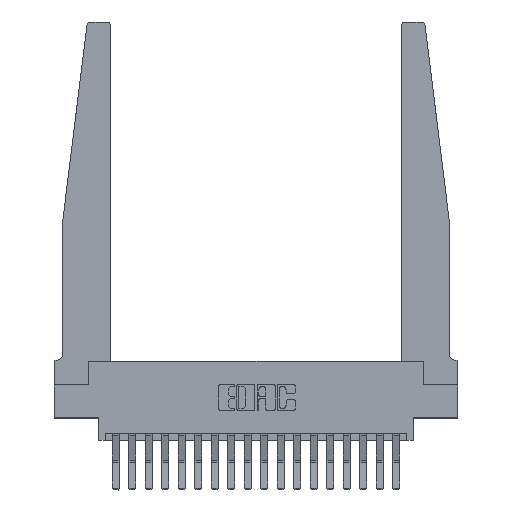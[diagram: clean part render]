
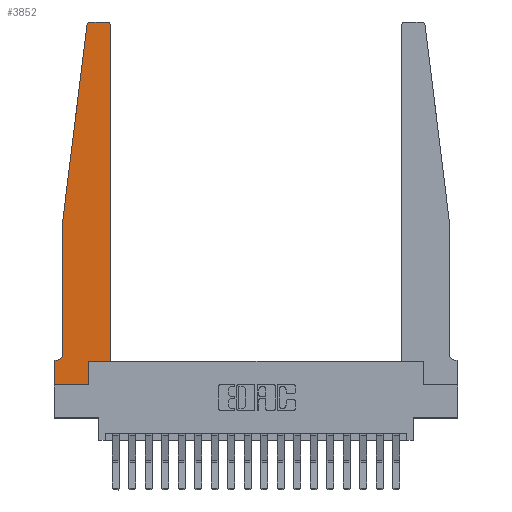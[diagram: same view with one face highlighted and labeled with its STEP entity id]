
A CAD part, top view. The second image highlights one B-rep face of the part: STEP entity #3852.
In plain terms, the highlighted planar face has unit normal (0, 0, 1).
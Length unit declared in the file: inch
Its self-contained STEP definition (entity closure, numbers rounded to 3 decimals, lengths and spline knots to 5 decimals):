
#74 = DIRECTION ( 'NONE',  ( 0., 1., 0. ) ) ;
#205 = DIRECTION ( 'NONE',  ( 0., 0., 1. ) ) ;
#353 = EDGE_LOOP ( 'NONE', ( #4655, #19632, #8052, #14852, #11743, #19731, #17841, #4805, #10594, #14451, #12872, #9959 ) ) ;
#477 = EDGE_CURVE ( 'NONE', #16946, #14493, #8638, .T. ) ;
#499 = CARTESIAN_POINT ( 'NONE',  ( 0.015, 0.2375, 0.37 ) ) ;
#650 = CIRCLE ( 'NONE', #15962, 0.03 ) ;
#971 = EDGE_CURVE ( 'NONE', #14493, #1321, #3538, .T. ) ;
#1109 = VECTOR ( 'NONE', #5097, 39.37008 ) ;
#1321 = VERTEX_POINT ( 'NONE', #9912 ) ;
#1363 = CARTESIAN_POINT ( 'NONE',  ( 0.065, 0.1875, 0.37 ) ) ;
#1855 = VECTOR ( 'NONE', #16621, 39.37008 ) ;
#2051 = DIRECTION ( 'NONE',  ( -1., 0., 0. ) ) ;
#2540 = CARTESIAN_POINT ( 'NONE',  ( 0., 0.1875, 0.37 ) ) ;
#3120 = CARTESIAN_POINT ( 'NONE',  ( 0.25, 2.75, 0.37 ) ) ;
#3167 = CARTESIAN_POINT ( 'NONE',  ( 0.425, 0.18, 0.37 ) ) ;
#3538 = CIRCLE ( 'NONE', #10757, 0.03 ) ;
#3852 = ADVANCED_FACE ( 'NONE', ( #19087 ), #6340, .T. ) ;
#3953 = CARTESIAN_POINT ( 'NONE',  ( 0., 0., 0.37 ) ) ;
#4562 = VERTEX_POINT ( 'NONE', #14441 ) ;
#4655 = ORIENTED_EDGE ( 'NONE', *, *, #477, .T. ) ;
#4674 = VECTOR ( 'NONE', #74, 39.37008 ) ;
#4805 = ORIENTED_EDGE ( 'NONE', *, *, #18043, .T. ) ;
#5097 = DIRECTION ( 'NONE',  ( 1., 0., 0. ) ) ;
#5315 = LINE ( 'NONE', #15316, #12548 ) ;
#5575 = DIRECTION ( 'NONE',  ( 0., 0., 1. ) ) ;
#5767 = DIRECTION ( 'NONE',  ( 0., -1., 0. ) ) ;
#5957 = LINE ( 'NONE', #7456, #1855 ) ;
#6118 = VECTOR ( 'NONE', #5767, 39.37008 ) ;
#6211 = VERTEX_POINT ( 'NONE', #19633 ) ;
#6285 = CARTESIAN_POINT ( 'NONE',  ( 0.2605, 0.18, 0.37 ) ) ;
#6340 = PLANE ( 'NONE',  #14887 ) ;
#6523 = VERTEX_POINT ( 'NONE', #9910 ) ;
#7456 = CARTESIAN_POINT ( 'NONE',  ( 0.425, 0.18, 0.37 ) ) ;
#7575 = DIRECTION ( 'NONE',  ( 0., 1., 0. ) ) ;
#8052 = ORIENTED_EDGE ( 'NONE', *, *, #11192, .T. ) ;
#8413 = VERTEX_POINT ( 'NONE', #6285 ) ;
#8549 = CIRCLE ( 'NONE', #12367, 0.05 ) ;
#8638 = LINE ( 'NONE', #3120, #16347 ) ;
#8852 = CARTESIAN_POINT ( 'NONE',  ( 0.27653, 2.75, 0.37 ) ) ;
#8969 = LINE ( 'NONE', #1363, #12093 ) ;
#9113 = CARTESIAN_POINT ( 'NONE',  ( 0.27653, 2.72, 0.37 ) ) ;
#9269 = EDGE_CURVE ( 'NONE', #13089, #16946, #650, .T. ) ;
#9309 = LINE ( 'NONE', #12846, #1109 ) ;
#9444 = CARTESIAN_POINT ( 'NONE',  ( 0., 0.1875, 0.37 ) ) ;
#9451 = EDGE_CURVE ( 'NONE', #8413, #13597, #5957, .T. ) ;
#9503 = VERTEX_POINT ( 'NONE', #15258 ) ;
#9910 = CARTESIAN_POINT ( 'NONE',  ( 0.015, 0.1875, 0.37 ) ) ;
#9912 = CARTESIAN_POINT ( 'NONE',  ( 0.24675, 2.72367, 0.37 ) ) ;
#9959 = ORIENTED_EDGE ( 'NONE', *, *, #9269, .T. ) ;
#10594 = ORIENTED_EDGE ( 'NONE', *, *, #13999, .T. ) ;
#10669 = DIRECTION ( 'NONE',  ( 1., 0., 0. ) ) ;
#10757 = AXIS2_PLACEMENT_3D ( 'NONE', #9113, #19903, #10669 ) ;
#10806 = EDGE_CURVE ( 'NONE', #4562, #6523, #8549, .T. ) ;
#10995 = DIRECTION ( 'NONE',  ( 1., 0., 0. ) ) ;
#11177 = CARTESIAN_POINT ( 'NONE',  ( 0.425, 0.18, 0.37 ) ) ;
#11192 = EDGE_CURVE ( 'NONE', #1321, #9503, #14539, .T. ) ;
#11294 = DIRECTION ( 'NONE',  ( 0., 0., -1. ) ) ;
#11642 = DIRECTION ( 'NONE',  ( 0., -1., 0. ) ) ;
#11743 = ORIENTED_EDGE ( 'NONE', *, *, #10806, .T. ) ;
#12093 = VECTOR ( 'NONE', #12159, 39.37008 ) ;
#12123 = EDGE_CURVE ( 'NONE', #18233, #6211, #19116, .T. ) ;
#12159 = DIRECTION ( 'NONE',  ( -1., 0., 0. ) ) ;
#12367 = AXIS2_PLACEMENT_3D ( 'NONE', #499, #11294, #2051 ) ;
#12548 = VECTOR ( 'NONE', #7575, 39.37008 ) ;
#12845 = EDGE_CURVE ( 'NONE', #6523, #18233, #8969, .T. ) ;
#12846 = CARTESIAN_POINT ( 'NONE',  ( 0., 0., 0.37 ) ) ;
#12872 = ORIENTED_EDGE ( 'NONE', *, *, #19077, .T. ) ;
#12927 = VERTEX_POINT ( 'NONE', #18480 ) ;
#13089 = VERTEX_POINT ( 'NONE', #14411 ) ;
#13597 = VERTEX_POINT ( 'NONE', #11177 ) ;
#13999 = EDGE_CURVE ( 'NONE', #12927, #8413, #5315, .T. ) ;
#14411 = CARTESIAN_POINT ( 'NONE',  ( 0.425, 2.72, 0.37 ) ) ;
#14441 = CARTESIAN_POINT ( 'NONE',  ( 0.065, 0.2375, 0.37 ) ) ;
#14451 = ORIENTED_EDGE ( 'NONE', *, *, #9451, .T. ) ;
#14493 = VERTEX_POINT ( 'NONE', #8852 ) ;
#14539 = LINE ( 'NONE', #18350, #15025 ) ;
#14793 = CARTESIAN_POINT ( 'NONE',  ( 0.395, 2.72, 0.37 ) ) ;
#14852 = ORIENTED_EDGE ( 'NONE', *, *, #19472, .T. ) ;
#14887 = AXIS2_PLACEMENT_3D ( 'NONE', #9444, #205, #10995 ) ;
#14970 = CARTESIAN_POINT ( 'NONE',  ( 0.065, 1.25, 0.37 ) ) ;
#14992 = VECTOR ( 'NONE', #11642, 39.37008 ) ;
#15025 = VECTOR ( 'NONE', #19909, 39.37008 ) ;
#15258 = CARTESIAN_POINT ( 'NONE',  ( 0.065, 1.25, 0.37 ) ) ;
#15316 = CARTESIAN_POINT ( 'NONE',  ( 0.2605, 0.18, 0.37 ) ) ;
#15962 = AXIS2_PLACEMENT_3D ( 'NONE', #14793, #5575, #16353 ) ;
#16256 = CARTESIAN_POINT ( 'NONE',  ( 0.395, 2.75, 0.37 ) ) ;
#16347 = VECTOR ( 'NONE', #17010, 39.37008 ) ;
#16353 = DIRECTION ( 'NONE',  ( 1., 0., 0. ) ) ;
#16502 = LINE ( 'NONE', #3167, #4674 ) ;
#16621 = DIRECTION ( 'NONE',  ( 1., 0., 0. ) ) ;
#16946 = VERTEX_POINT ( 'NONE', #16256 ) ;
#17010 = DIRECTION ( 'NONE',  ( -1., 0., 0. ) ) ;
#17841 = ORIENTED_EDGE ( 'NONE', *, *, #12123, .T. ) ;
#17939 = LINE ( 'NONE', #14970, #6118 ) ;
#18043 = EDGE_CURVE ( 'NONE', #6211, #12927, #9309, .T. ) ;
#18233 = VERTEX_POINT ( 'NONE', #2540 ) ;
#18350 = CARTESIAN_POINT ( 'NONE',  ( 0.065, 1.25, 0.37 ) ) ;
#18480 = CARTESIAN_POINT ( 'NONE',  ( 0.2605, 0., 0.37 ) ) ;
#19077 = EDGE_CURVE ( 'NONE', #13597, #13089, #16502, .T. ) ;
#19087 = FACE_OUTER_BOUND ( 'NONE', #353, .T. ) ;
#19116 = LINE ( 'NONE', #3953, #14992 ) ;
#19472 = EDGE_CURVE ( 'NONE', #9503, #4562, #17939, .T. ) ;
#19632 = ORIENTED_EDGE ( 'NONE', *, *, #971, .T. ) ;
#19633 = CARTESIAN_POINT ( 'NONE',  ( 0., 0., 0.37 ) ) ;
#19731 = ORIENTED_EDGE ( 'NONE', *, *, #12845, .T. ) ;
#19903 = DIRECTION ( 'NONE',  ( 0., 0., 1. ) ) ;
#19909 = DIRECTION ( 'NONE',  ( -0.122, -0.992, 0. ) ) ;
